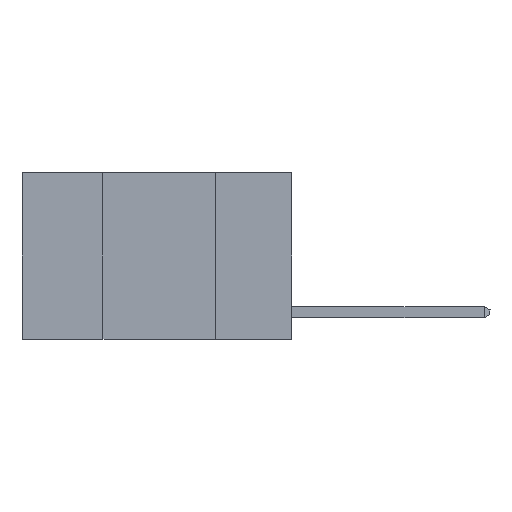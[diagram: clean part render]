
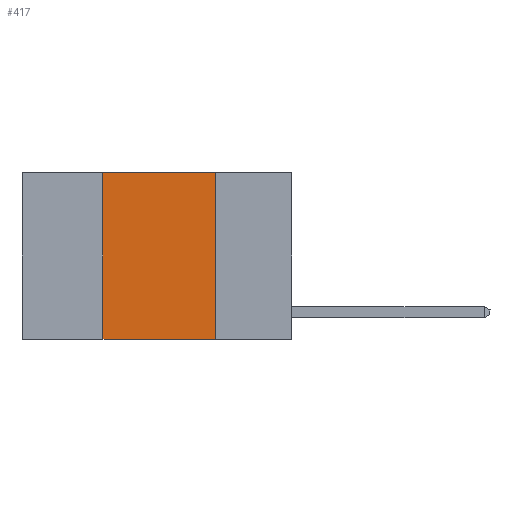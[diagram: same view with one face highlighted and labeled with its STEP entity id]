
A CAD part, left-side view. The second image highlights one B-rep face of the part: STEP entity #417.
In plain terms, the highlighted planar face has unit normal (-1, 0, 0).
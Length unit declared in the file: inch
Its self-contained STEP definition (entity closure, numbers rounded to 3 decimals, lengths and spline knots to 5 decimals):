
#417 = ADVANCED_FACE ( 'NONE', ( #1566 ), #16401, .F. ) ;
#517 = EDGE_CURVE ( 'NONE', #4201, #3305, #16166, .T. ) ;
#1083 = CARTESIAN_POINT ( 'NONE',  ( 0., 0.17, 0. ) ) ;
#1229 = VECTOR ( 'NONE', #16836, 39.37008 ) ;
#1344 = CARTESIAN_POINT ( 'NONE',  ( 0., 0.6, 0. ) ) ;
#1566 = FACE_OUTER_BOUND ( 'NONE', #14000, .T. ) ;
#1571 = EDGE_CURVE ( 'NONE', #4772, #11783, #3544, .T. ) ;
#1911 = DIRECTION ( 'NONE',  ( 0., 0., -1. ) ) ;
#2301 = ORIENTED_EDGE ( 'NONE', *, *, #517, .F. ) ;
#2582 = VECTOR ( 'NONE', #3908, 39.37008 ) ;
#2650 = EDGE_CURVE ( 'NONE', #4772, #3305, #12605, .T. ) ;
#2767 = DIRECTION ( 'NONE',  ( 0., -1., 0. ) ) ;
#3156 = DIRECTION ( 'NONE',  ( 1., 0., 0. ) ) ;
#3305 = VERTEX_POINT ( 'NONE', #12033 ) ;
#3544 = LINE ( 'NONE', #15305, #7527 ) ;
#3908 = DIRECTION ( 'NONE',  ( 0., 0., -1. ) ) ;
#4201 = VERTEX_POINT ( 'NONE', #8210 ) ;
#4344 = ORIENTED_EDGE ( 'NONE', *, *, #1571, .F. ) ;
#4772 = VERTEX_POINT ( 'NONE', #15310 ) ;
#5701 = ORIENTED_EDGE ( 'NONE', *, *, #2650, .T. ) ;
#5744 = LINE ( 'NONE', #1344, #16614 ) ;
#7173 = AXIS2_PLACEMENT_3D ( 'NONE', #17047, #3156, #1911 ) ;
#7527 = VECTOR ( 'NONE', #13562, 39.37008 ) ;
#8210 = CARTESIAN_POINT ( 'NONE',  ( 0., 0.17, 0. ) ) ;
#11783 = VERTEX_POINT ( 'NONE', #15371 ) ;
#12033 = CARTESIAN_POINT ( 'NONE',  ( 0., 0.17, -0.37 ) ) ;
#12350 = ORIENTED_EDGE ( 'NONE', *, *, #15000, .F. ) ;
#12605 = LINE ( 'NONE', #13997, #1229 ) ;
#13562 = DIRECTION ( 'NONE',  ( 0., 0., 1. ) ) ;
#13997 = CARTESIAN_POINT ( 'NONE',  ( 0., 0.6, -0.37 ) ) ;
#14000 = EDGE_LOOP ( 'NONE', ( #2301, #12350, #4344, #5701 ) ) ;
#15000 = EDGE_CURVE ( 'NONE', #11783, #4201, #5744, .T. ) ;
#15305 = CARTESIAN_POINT ( 'NONE',  ( 0., 0.42, 0. ) ) ;
#15310 = CARTESIAN_POINT ( 'NONE',  ( 0., 0.42, -0.37 ) ) ;
#15371 = CARTESIAN_POINT ( 'NONE',  ( 0., 0.42, 0. ) ) ;
#16166 = LINE ( 'NONE', #1083, #2582 ) ;
#16401 = PLANE ( 'NONE',  #7173 ) ;
#16614 = VECTOR ( 'NONE', #2767, 39.37008 ) ;
#16836 = DIRECTION ( 'NONE',  ( 0., -1., 0. ) ) ;
#17047 = CARTESIAN_POINT ( 'NONE',  ( 0., 0.6, 0. ) ) ;
